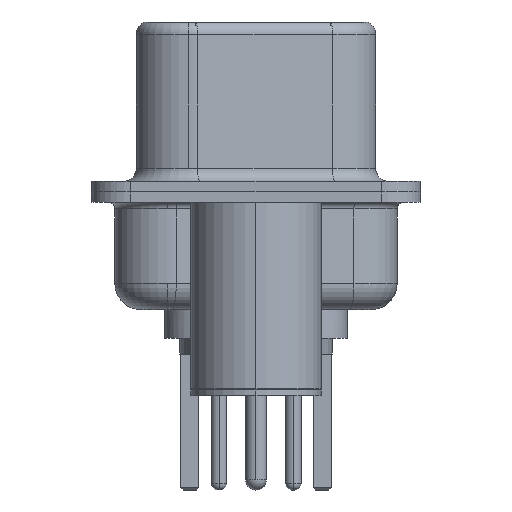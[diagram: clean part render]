
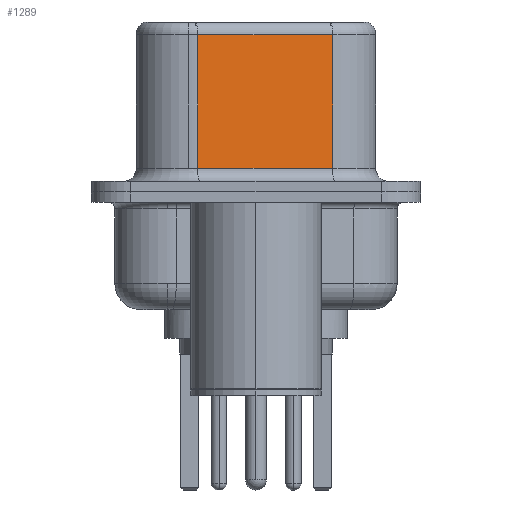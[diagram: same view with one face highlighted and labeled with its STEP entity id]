
A CAD part, left-side view. The second image highlights one B-rep face of the part: STEP entity #1289.
In plain terms, the highlighted planar face has unit normal (-0.985, -0.174, 0).
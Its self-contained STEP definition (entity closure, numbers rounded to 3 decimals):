
#554 = LINE ( 'NONE', #980, #10591 ) ;
#980 = CARTESIAN_POINT ( 'NONE',  ( 3.67, 2.233, 6.52 ) ) ;
#1277 = CARTESIAN_POINT ( 'NONE',  ( 4.58, -2.927, 0.9 ) ) ;
#1289 = ADVANCED_FACE ( 'NONE', ( #3923 ), #24589, .F. ) ;
#1445 = CARTESIAN_POINT ( 'NONE',  ( 4.58, -2.927, 0.9 ) ) ;
#3117 = VERTEX_POINT ( 'NONE', #15951 ) ;
#3923 = FACE_OUTER_BOUND ( 'NONE', #5216, .T. ) ;
#4390 = EDGE_CURVE ( 'NONE', #13816, #3117, #554, .T. ) ;
#4766 = CARTESIAN_POINT ( 'NONE',  ( 4.58, -2.927, 6.02 ) ) ;
#5216 = EDGE_LOOP ( 'NONE', ( #6809, #22282, #23336, #15866 ) ) ;
#5915 = VECTOR ( 'NONE', #14499, 1000. ) ;
#6809 = ORIENTED_EDGE ( 'NONE', *, *, #22789, .F. ) ;
#9665 = VERTEX_POINT ( 'NONE', #4766 ) ;
#9674 = VECTOR ( 'NONE', #11163, 1000. ) ;
#10313 = DIRECTION ( 'NONE',  ( 0.985, 0.174, 0. ) ) ;
#10591 = VECTOR ( 'NONE', #12314, 1000. ) ;
#11163 = DIRECTION ( 'NONE',  ( 0., 0., -1. ) ) ;
#12314 = DIRECTION ( 'NONE',  ( 0., 0., -1. ) ) ;
#13504 = AXIS2_PLACEMENT_3D ( 'NONE', #17416, #10313, #17264 ) ;
#13816 = VERTEX_POINT ( 'NONE', #19617 ) ;
#14499 = DIRECTION ( 'NONE',  ( -0.174, 0.985, 0. ) ) ;
#14589 = EDGE_CURVE ( 'NONE', #9665, #13816, #15273, .T. ) ;
#15273 = LINE ( 'NONE', #18518, #5915 ) ;
#15866 = ORIENTED_EDGE ( 'NONE', *, *, #16294, .T. ) ;
#15951 = CARTESIAN_POINT ( 'NONE',  ( 3.67, 2.233, 0.9 ) ) ;
#16294 = EDGE_CURVE ( 'NONE', #3117, #22903, #23671, .T. ) ;
#17085 = CARTESIAN_POINT ( 'NONE',  ( 4.58, -2.927, 6.52 ) ) ;
#17264 = DIRECTION ( 'NONE',  ( -0.174, 0.985, 0. ) ) ;
#17416 = CARTESIAN_POINT ( 'NONE',  ( 4.58, -2.927, 6.52 ) ) ;
#18353 = VECTOR ( 'NONE', #21173, 1000. ) ;
#18518 = CARTESIAN_POINT ( 'NONE',  ( 4.58, -2.927, 6.02 ) ) ;
#19617 = CARTESIAN_POINT ( 'NONE',  ( 3.67, 2.233, 6.02 ) ) ;
#20246 = LINE ( 'NONE', #17085, #9674 ) ;
#21173 = DIRECTION ( 'NONE',  ( 0.174, -0.985, 0. ) ) ;
#22282 = ORIENTED_EDGE ( 'NONE', *, *, #14589, .T. ) ;
#22789 = EDGE_CURVE ( 'NONE', #9665, #22903, #20246, .T. ) ;
#22903 = VERTEX_POINT ( 'NONE', #1445 ) ;
#23336 = ORIENTED_EDGE ( 'NONE', *, *, #4390, .T. ) ;
#23671 = LINE ( 'NONE', #1277, #18353 ) ;
#24589 = PLANE ( 'NONE',  #13504 ) ;
